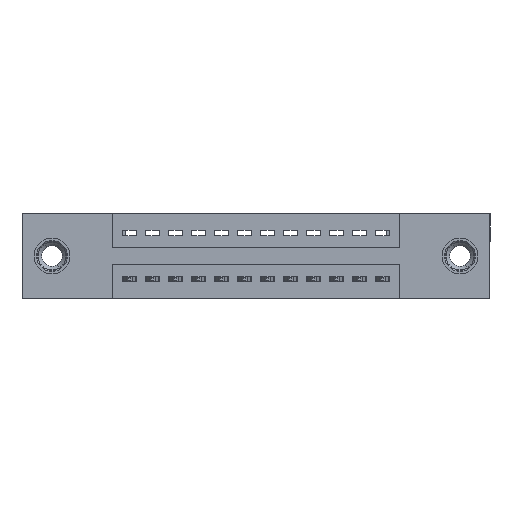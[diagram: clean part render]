
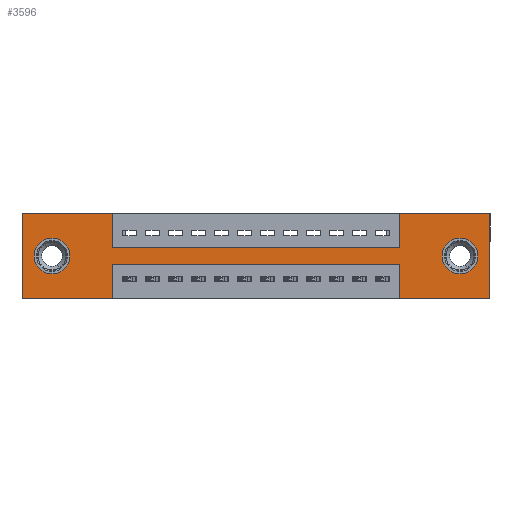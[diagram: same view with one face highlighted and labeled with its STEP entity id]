
A CAD part, front view. The second image highlights one B-rep face of the part: STEP entity #3596.
In plain terms, the highlighted planar face has unit normal (0, -1, 0).
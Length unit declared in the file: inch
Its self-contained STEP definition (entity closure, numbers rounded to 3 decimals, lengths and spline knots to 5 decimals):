
#8 = DIRECTION ( 'NONE',  ( 0., 0., -1. ) ) ;
#26 = CARTESIAN_POINT ( 'NONE',  ( 2.035, 0., 0. ) ) ;
#151 = DIRECTION ( 'NONE',  ( 0., 1., 0. ) ) ;
#412 = EDGE_CURVE ( 'NONE', #7116, #16620, #585, .T. ) ;
#526 = CARTESIAN_POINT ( 'NONE',  ( 0.3925, 0., -0.22 ) ) ;
#571 = VERTEX_POINT ( 'NONE', #526 ) ;
#585 = LINE ( 'NONE', #7707, #14818 ) ;
#663 = CARTESIAN_POINT ( 'NONE',  ( 0.13, 0., -0.185 ) ) ;
#1417 = EDGE_CURVE ( 'NONE', #571, #7116, #9685, .T. ) ;
#1576 = LINE ( 'NONE', #6371, #3942 ) ;
#1641 = VERTEX_POINT ( 'NONE', #6306 ) ;
#1645 = CARTESIAN_POINT ( 'NONE',  ( 0.13, 0., -0.263 ) ) ;
#1829 = VECTOR ( 'NONE', #9158, 39.37008 ) ;
#1844 = DIRECTION ( 'NONE',  ( 0., 1., 0. ) ) ;
#1881 = VERTEX_POINT ( 'NONE', #2628 ) ;
#1904 = CARTESIAN_POINT ( 'NONE',  ( 0., 0., -0.37 ) ) ;
#1906 = DIRECTION ( 'NONE',  ( 0., 0., 1. ) ) ;
#2031 = LINE ( 'NONE', #11718, #15355 ) ;
#2260 = VECTOR ( 'NONE', #13192, 39.37008 ) ;
#2265 = PLANE ( 'NONE',  #6498 ) ;
#2628 = CARTESIAN_POINT ( 'NONE',  ( 0.13, 0., -0.107 ) ) ;
#2697 = LINE ( 'NONE', #9359, #1829 ) ;
#3116 = EDGE_CURVE ( 'NONE', #8838, #16217, #16446, .T. ) ;
#3127 = LINE ( 'NONE', #17383, #2260 ) ;
#3160 = CARTESIAN_POINT ( 'NONE',  ( 0.3925, 0., -0.22 ) ) ;
#3200 = CARTESIAN_POINT ( 'NONE',  ( 1.6425, 0., -0.37 ) ) ;
#3203 = VECTOR ( 'NONE', #8, 39.37008 ) ;
#3233 = ORIENTED_EDGE ( 'NONE', *, *, #9673, .F. ) ;
#3596 = ADVANCED_FACE ( 'NONE', ( #8305, #4182, #3962 ), #2265, .T. ) ;
#3869 = ORIENTED_EDGE ( 'NONE', *, *, #14874, .F. ) ;
#3891 = CARTESIAN_POINT ( 'NONE',  ( 2.035, 0., 0. ) ) ;
#3942 = VECTOR ( 'NONE', #10563, 39.37008 ) ;
#3962 = FACE_OUTER_BOUND ( 'NONE', #5485, .T. ) ;
#4148 = CARTESIAN_POINT ( 'NONE',  ( 0.3925, 0., -0.37 ) ) ;
#4182 = FACE_BOUND ( 'NONE', #16175, .T. ) ;
#4409 = VERTEX_POINT ( 'NONE', #3200 ) ;
#4524 = EDGE_CURVE ( 'NONE', #11558, #1881, #14071, .T. ) ;
#4744 = ORIENTED_EDGE ( 'NONE', *, *, #4524, .T. ) ;
#4948 = ORIENTED_EDGE ( 'NONE', *, *, #3116, .F. ) ;
#5054 = CARTESIAN_POINT ( 'NONE',  ( 1.905, 0., -0.185 ) ) ;
#5061 = DIRECTION ( 'NONE',  ( 0., 0., -1. ) ) ;
#5125 = CARTESIAN_POINT ( 'NONE',  ( 0., 0., -0.37 ) ) ;
#5140 = DIRECTION ( 'NONE',  ( 1., 0., 0. ) ) ;
#5227 = CARTESIAN_POINT ( 'NONE',  ( 1.6425, 0., -0.37 ) ) ;
#5281 = DIRECTION ( 'NONE',  ( 0., 0., 1. ) ) ;
#5302 = VERTEX_POINT ( 'NONE', #14728 ) ;
#5363 = LINE ( 'NONE', #3160, #9725 ) ;
#5485 = EDGE_LOOP ( 'NONE', ( #15463, #7519, #11293, #7904, #3869, #4948, #15948, #6447, #3233, #9026, #15944, #15883 ) ) ;
#5589 = ORIENTED_EDGE ( 'NONE', *, *, #6694, .T. ) ;
#5982 = CIRCLE ( 'NONE', #14714, 0.078 ) ;
#6233 = VERTEX_POINT ( 'NONE', #13527 ) ;
#6258 = DIRECTION ( 'NONE',  ( -1., 0., 0. ) ) ;
#6306 = CARTESIAN_POINT ( 'NONE',  ( 0., 0., 0. ) ) ;
#6310 = CARTESIAN_POINT ( 'NONE',  ( 0., 0., 0. ) ) ;
#6325 = VECTOR ( 'NONE', #8211, 39.37008 ) ;
#6371 = CARTESIAN_POINT ( 'NONE',  ( 0.3925, 0., 0. ) ) ;
#6394 = DIRECTION ( 'NONE',  ( 0., 0., -1. ) ) ;
#6447 = ORIENTED_EDGE ( 'NONE', *, *, #8678, .F. ) ;
#6498 = AXIS2_PLACEMENT_3D ( 'NONE', #5125, #13321, #5061 ) ;
#6570 = ORIENTED_EDGE ( 'NONE', *, *, #12765, .T. ) ;
#6694 = EDGE_CURVE ( 'NONE', #11198, #5302, #15198, .T. ) ;
#6774 = DIRECTION ( 'NONE',  ( 0., 0., -1. ) ) ;
#7116 = VERTEX_POINT ( 'NONE', #4148 ) ;
#7519 = ORIENTED_EDGE ( 'NONE', *, *, #15239, .F. ) ;
#7524 = DIRECTION ( 'NONE',  ( 0., 1., 0. ) ) ;
#7637 = DIRECTION ( 'NONE',  ( 0., 0., 1. ) ) ;
#7701 = DIRECTION ( 'NONE',  ( 1., 0., 0. ) ) ;
#7707 = CARTESIAN_POINT ( 'NONE',  ( 0., 0., -0.37 ) ) ;
#7819 = CARTESIAN_POINT ( 'NONE',  ( 0., 0., 0. ) ) ;
#7904 = ORIENTED_EDGE ( 'NONE', *, *, #12745, .F. ) ;
#8211 = DIRECTION ( 'NONE',  ( 0., 0., 1. ) ) ;
#8305 = FACE_BOUND ( 'NONE', #10130, .T. ) ;
#8528 = EDGE_CURVE ( 'NONE', #1641, #6233, #14751, .T. ) ;
#8534 = CARTESIAN_POINT ( 'NONE',  ( 1.905, 0., -0.107 ) ) ;
#8615 = CARTESIAN_POINT ( 'NONE',  ( 1.6425, 0., -0.15 ) ) ;
#8678 = EDGE_CURVE ( 'NONE', #8734, #10910, #2697, .T. ) ;
#8703 = VECTOR ( 'NONE', #5281, 39.37008 ) ;
#8734 = VERTEX_POINT ( 'NONE', #10971 ) ;
#8838 = VERTEX_POINT ( 'NONE', #9174 ) ;
#9026 = ORIENTED_EDGE ( 'NONE', *, *, #8528, .F. ) ;
#9087 = DIRECTION ( 'NONE',  ( 0., 1., 0. ) ) ;
#9158 = DIRECTION ( 'NONE',  ( 1., 0., 0. ) ) ;
#9174 = CARTESIAN_POINT ( 'NONE',  ( 1.6425, 0., 0. ) ) ;
#9359 = CARTESIAN_POINT ( 'NONE',  ( 0.3925, 0., -0.15 ) ) ;
#9371 = LINE ( 'NONE', #15216, #6325 ) ;
#9673 = EDGE_CURVE ( 'NONE', #6233, #8734, #1576, .T. ) ;
#9685 = LINE ( 'NONE', #9839, #3203 ) ;
#9725 = VECTOR ( 'NONE', #16780, 39.37008 ) ;
#9732 = VERTEX_POINT ( 'NONE', #13007 ) ;
#9798 = AXIS2_PLACEMENT_3D ( 'NONE', #5054, #9087, #6394 ) ;
#9805 = CARTESIAN_POINT ( 'NONE',  ( 1.905, 0., -0.185 ) ) ;
#9839 = CARTESIAN_POINT ( 'NONE',  ( 0.3925, 0., -0.37 ) ) ;
#10083 = EDGE_CURVE ( 'NONE', #4409, #13167, #13612, .T. ) ;
#10130 = EDGE_LOOP ( 'NONE', ( #5589, #6570 ) ) ;
#10563 = DIRECTION ( 'NONE',  ( 0., 0., -1. ) ) ;
#10910 = VERTEX_POINT ( 'NONE', #8615 ) ;
#10971 = CARTESIAN_POINT ( 'NONE',  ( 0.3925, 0., -0.15 ) ) ;
#11198 = VERTEX_POINT ( 'NONE', #8534 ) ;
#11293 = ORIENTED_EDGE ( 'NONE', *, *, #10083, .F. ) ;
#11558 = VERTEX_POINT ( 'NONE', #1645 ) ;
#11718 = CARTESIAN_POINT ( 'NONE',  ( 0., 0., 0. ) ) ;
#12510 = LINE ( 'NONE', #26, #13163 ) ;
#12745 = EDGE_CURVE ( 'NONE', #9732, #4409, #3127, .T. ) ;
#12765 = EDGE_CURVE ( 'NONE', #5302, #11198, #15117, .T. ) ;
#13007 = CARTESIAN_POINT ( 'NONE',  ( 2.035, 0., -0.37 ) ) ;
#13030 = EDGE_CURVE ( 'NONE', #16620, #1641, #2031, .T. ) ;
#13163 = VECTOR ( 'NONE', #6774, 39.37008 ) ;
#13167 = VERTEX_POINT ( 'NONE', #15889 ) ;
#13192 = DIRECTION ( 'NONE',  ( -1., 0., 0. ) ) ;
#13321 = DIRECTION ( 'NONE',  ( 0., -1., 0. ) ) ;
#13527 = CARTESIAN_POINT ( 'NONE',  ( 0.3925, 0., 0. ) ) ;
#13562 = EDGE_CURVE ( 'NONE', #10910, #8838, #9371, .T. ) ;
#13612 = LINE ( 'NONE', #5227, #8703 ) ;
#13974 = AXIS2_PLACEMENT_3D ( 'NONE', #9805, #151, #15329 ) ;
#14071 = CIRCLE ( 'NONE', #17428, 0.078 ) ;
#14324 = VECTOR ( 'NONE', #5140, 39.37008 ) ;
#14714 = AXIS2_PLACEMENT_3D ( 'NONE', #16856, #1844, #15545 ) ;
#14728 = CARTESIAN_POINT ( 'NONE',  ( 1.905, 0., -0.263 ) ) ;
#14751 = LINE ( 'NONE', #7819, #14324 ) ;
#14755 = VECTOR ( 'NONE', #7701, 39.37008 ) ;
#14818 = VECTOR ( 'NONE', #6258, 39.37008 ) ;
#14874 = EDGE_CURVE ( 'NONE', #16217, #9732, #12510, .T. ) ;
#15117 = CIRCLE ( 'NONE', #13974, 0.078 ) ;
#15198 = CIRCLE ( 'NONE', #9798, 0.078 ) ;
#15216 = CARTESIAN_POINT ( 'NONE',  ( 1.6425, 0., 0. ) ) ;
#15239 = EDGE_CURVE ( 'NONE', #13167, #571, #5363, .T. ) ;
#15329 = DIRECTION ( 'NONE',  ( 0., 0., -1. ) ) ;
#15355 = VECTOR ( 'NONE', #1906, 39.37008 ) ;
#15463 = ORIENTED_EDGE ( 'NONE', *, *, #1417, .F. ) ;
#15545 = DIRECTION ( 'NONE',  ( 0., 0., 1. ) ) ;
#15883 = ORIENTED_EDGE ( 'NONE', *, *, #412, .F. ) ;
#15889 = CARTESIAN_POINT ( 'NONE',  ( 1.6425, 0., -0.22 ) ) ;
#15943 = ORIENTED_EDGE ( 'NONE', *, *, #16669, .T. ) ;
#15944 = ORIENTED_EDGE ( 'NONE', *, *, #13030, .F. ) ;
#15948 = ORIENTED_EDGE ( 'NONE', *, *, #13562, .F. ) ;
#16175 = EDGE_LOOP ( 'NONE', ( #15943, #4744 ) ) ;
#16217 = VERTEX_POINT ( 'NONE', #3891 ) ;
#16446 = LINE ( 'NONE', #6310, #14755 ) ;
#16620 = VERTEX_POINT ( 'NONE', #1904 ) ;
#16669 = EDGE_CURVE ( 'NONE', #1881, #11558, #5982, .T. ) ;
#16780 = DIRECTION ( 'NONE',  ( -1., 0., 0. ) ) ;
#16856 = CARTESIAN_POINT ( 'NONE',  ( 0.13, 0., -0.185 ) ) ;
#17383 = CARTESIAN_POINT ( 'NONE',  ( 0., 0., -0.37 ) ) ;
#17428 = AXIS2_PLACEMENT_3D ( 'NONE', #663, #7524, #7637 ) ;
